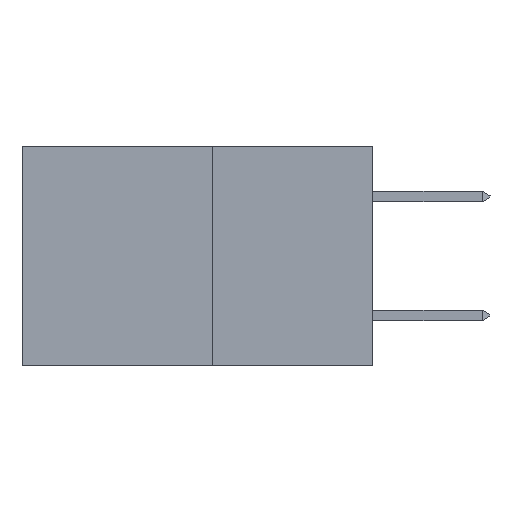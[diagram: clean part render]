
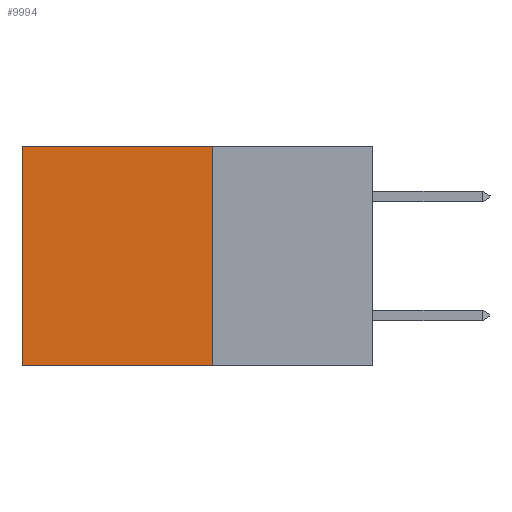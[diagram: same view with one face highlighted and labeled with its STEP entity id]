
A CAD part, left-side view. The second image highlights one B-rep face of the part: STEP entity #9994.
In plain terms, the highlighted planar face has unit normal (-1, 0, 0).
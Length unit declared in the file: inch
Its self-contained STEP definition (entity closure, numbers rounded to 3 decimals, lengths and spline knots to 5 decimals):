
#1 = AXIS2_PLACEMENT_3D ( 'NONE', #5066, #27044, #13680 ) ;
#530 = ORIENTED_EDGE ( 'NONE', *, *, #6680, .T. ) ;
#3521 = ORIENTED_EDGE ( 'NONE', *, *, #21180, .F. ) ;
#4030 = VERTEX_POINT ( 'NONE', #8760 ) ;
#4063 = LINE ( 'NONE', #28082, #14815 ) ;
#4302 = VECTOR ( 'NONE', #17382, 39.37008 ) ;
#5066 = CARTESIAN_POINT ( 'NONE',  ( 0.277, 0.27, -0.37 ) ) ;
#6015 = DIRECTION ( 'NONE',  ( 0., 1., 0. ) ) ;
#6453 = DIRECTION ( 'NONE',  ( 0., 0., -1. ) ) ;
#6680 = EDGE_CURVE ( 'NONE', #7838, #6704, #15063, .T. ) ;
#6704 = VERTEX_POINT ( 'NONE', #23988 ) ;
#7496 = CARTESIAN_POINT ( 'NONE',  ( 0.277, 0.27, -0.37 ) ) ;
#7838 = VERTEX_POINT ( 'NONE', #17896 ) ;
#8193 = CARTESIAN_POINT ( 'NONE',  ( 0.277, 0.27, -0.37 ) ) ;
#8224 = VERTEX_POINT ( 'NONE', #8193 ) ;
#8760 = CARTESIAN_POINT ( 'NONE',  ( 0.277, 0.59, -0.37 ) ) ;
#8765 = EDGE_CURVE ( 'NONE', #7838, #8224, #23436, .T. ) ;
#9994 = ADVANCED_FACE ( 'NONE', ( #23718 ), #24793, .F. ) ;
#10775 = EDGE_LOOP ( 'NONE', ( #12880, #3521, #22987, #530 ) ) ;
#11621 = VECTOR ( 'NONE', #27264, 39.37008 ) ;
#12880 = ORIENTED_EDGE ( 'NONE', *, *, #14045, .T. ) ;
#13680 = DIRECTION ( 'NONE',  ( 0., 0., -1. ) ) ;
#14045 = EDGE_CURVE ( 'NONE', #6704, #4030, #14442, .T. ) ;
#14442 = LINE ( 'NONE', #15022, #19721 ) ;
#14815 = VECTOR ( 'NONE', #6015, 39.37008 ) ;
#15022 = CARTESIAN_POINT ( 'NONE',  ( 0.277, 0.59, -0.37 ) ) ;
#15063 = LINE ( 'NONE', #17347, #4302 ) ;
#17347 = CARTESIAN_POINT ( 'NONE',  ( 0.277, 0.27, 0. ) ) ;
#17382 = DIRECTION ( 'NONE',  ( 0., 1., 0. ) ) ;
#17896 = CARTESIAN_POINT ( 'NONE',  ( 0.277, 0.27, 0. ) ) ;
#19721 = VECTOR ( 'NONE', #6453, 39.37008 ) ;
#21180 = EDGE_CURVE ( 'NONE', #8224, #4030, #4063, .T. ) ;
#22987 = ORIENTED_EDGE ( 'NONE', *, *, #8765, .F. ) ;
#23436 = LINE ( 'NONE', #7496, #11621 ) ;
#23718 = FACE_OUTER_BOUND ( 'NONE', #10775, .T. ) ;
#23988 = CARTESIAN_POINT ( 'NONE',  ( 0.277, 0.59, 0. ) ) ;
#24793 = PLANE ( 'NONE',  #1 ) ;
#27044 = DIRECTION ( 'NONE',  ( 1., 0., 0. ) ) ;
#27264 = DIRECTION ( 'NONE',  ( 0., 0., -1. ) ) ;
#28082 = CARTESIAN_POINT ( 'NONE',  ( 0.277, 0.27, -0.37 ) ) ;
